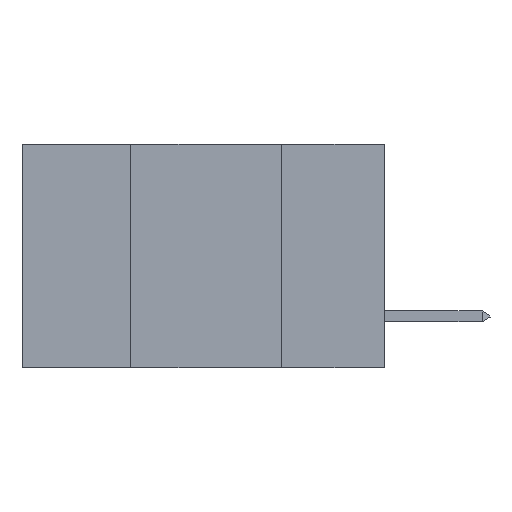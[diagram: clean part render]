
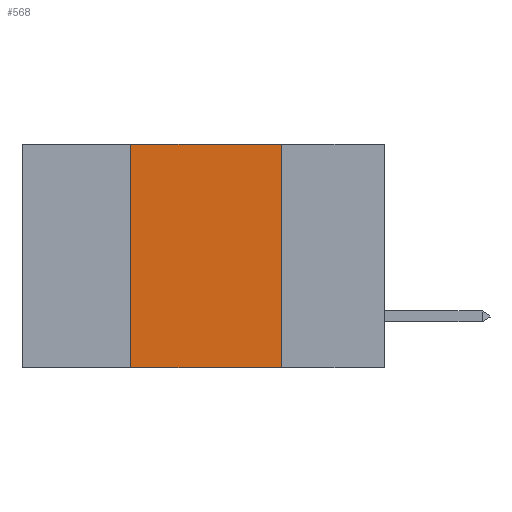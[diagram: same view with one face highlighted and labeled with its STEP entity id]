
A CAD part, left-side view. The second image highlights one B-rep face of the part: STEP entity #568.
In plain terms, the highlighted planar face has unit normal (-1, 0, 0).
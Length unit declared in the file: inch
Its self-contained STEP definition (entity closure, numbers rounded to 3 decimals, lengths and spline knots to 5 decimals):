
#568 = ADVANCED_FACE ( 'NONE', ( #9292 ), #5329, .F. ) ;
#1002 = CARTESIAN_POINT ( 'NONE',  ( 0., 0.17, 0. ) ) ;
#1574 = CARTESIAN_POINT ( 'NONE',  ( 0., 0.17, -0.37 ) ) ;
#1723 = ORIENTED_EDGE ( 'NONE', *, *, #7527, .F. ) ;
#2617 = LINE ( 'NONE', #6133, #9635 ) ;
#2824 = CARTESIAN_POINT ( 'NONE',  ( 0., 0.17, 0. ) ) ;
#3214 = DIRECTION ( 'NONE',  ( 0., 0., -1. ) ) ;
#3391 = VERTEX_POINT ( 'NONE', #3480 ) ;
#3480 = CARTESIAN_POINT ( 'NONE',  ( 0., 0.42, 0. ) ) ;
#3495 = DIRECTION ( 'NONE',  ( 0., 0., 1. ) ) ;
#4479 = ORIENTED_EDGE ( 'NONE', *, *, #5924, .F. ) ;
#4900 = CARTESIAN_POINT ( 'NONE',  ( 0., 0.6, 0. ) ) ;
#5119 = VECTOR ( 'NONE', #15877, 39.37008 ) ;
#5250 = VERTEX_POINT ( 'NONE', #15090 ) ;
#5329 = PLANE ( 'NONE',  #9492 ) ;
#5924 = EDGE_CURVE ( 'NONE', #3391, #15544, #9452, .T. ) ;
#6133 = CARTESIAN_POINT ( 'NONE',  ( 0., 0.42, 0. ) ) ;
#7267 = EDGE_LOOP ( 'NONE', ( #17857, #4479, #1723, #14991 ) ) ;
#7318 = DIRECTION ( 'NONE',  ( 1., 0., 0. ) ) ;
#7372 = DIRECTION ( 'NONE',  ( 0., -1., 0. ) ) ;
#7527 = EDGE_CURVE ( 'NONE', #5250, #3391, #2617, .T. ) ;
#7609 = LINE ( 'NONE', #2824, #5119 ) ;
#9292 = FACE_OUTER_BOUND ( 'NONE', #7267, .T. ) ;
#9452 = LINE ( 'NONE', #4900, #11517 ) ;
#9492 = AXIS2_PLACEMENT_3D ( 'NONE', #14612, #7318, #3214 ) ;
#9635 = VECTOR ( 'NONE', #3495, 39.37008 ) ;
#11517 = VECTOR ( 'NONE', #18048, 39.37008 ) ;
#14612 = CARTESIAN_POINT ( 'NONE',  ( 0., 0.6, 0. ) ) ;
#14991 = ORIENTED_EDGE ( 'NONE', *, *, #18495, .T. ) ;
#15046 = EDGE_CURVE ( 'NONE', #15544, #15699, #7609, .T. ) ;
#15090 = CARTESIAN_POINT ( 'NONE',  ( 0., 0.42, -0.37 ) ) ;
#15544 = VERTEX_POINT ( 'NONE', #1002 ) ;
#15660 = VECTOR ( 'NONE', #7372, 39.37008 ) ;
#15699 = VERTEX_POINT ( 'NONE', #1574 ) ;
#15877 = DIRECTION ( 'NONE',  ( 0., 0., -1. ) ) ;
#15886 = CARTESIAN_POINT ( 'NONE',  ( 0., 0.6, -0.37 ) ) ;
#17857 = ORIENTED_EDGE ( 'NONE', *, *, #15046, .F. ) ;
#17954 = LINE ( 'NONE', #15886, #15660 ) ;
#18048 = DIRECTION ( 'NONE',  ( 0., -1., 0. ) ) ;
#18495 = EDGE_CURVE ( 'NONE', #5250, #15699, #17954, .T. ) ;
